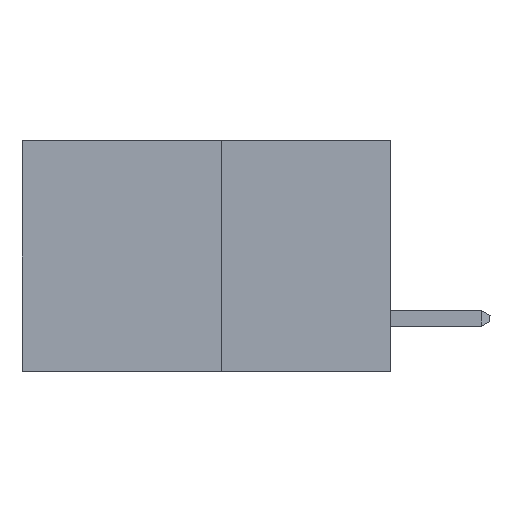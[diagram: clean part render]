
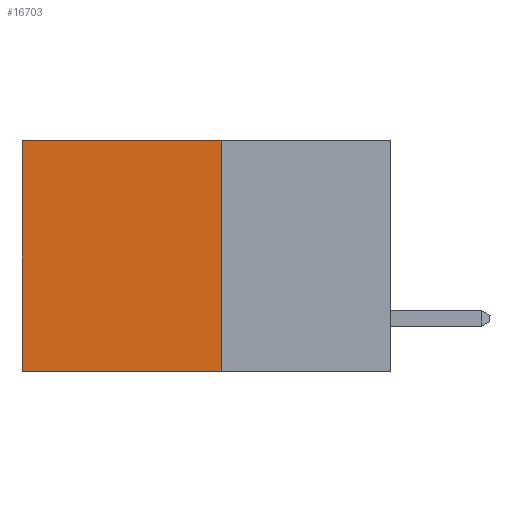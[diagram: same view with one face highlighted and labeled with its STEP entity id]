
A CAD part, left-side view. The second image highlights one B-rep face of the part: STEP entity #16703.
In plain terms, the highlighted planar face has unit normal (-1, 0, 0).
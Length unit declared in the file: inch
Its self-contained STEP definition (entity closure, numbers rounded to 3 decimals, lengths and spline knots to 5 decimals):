
#2117 = AXIS2_PLACEMENT_3D ( 'NONE', #9706, #24989, #11933 ) ;
#3600 = DIRECTION ( 'NONE',  ( 0., 1., 0. ) ) ;
#6845 = DIRECTION ( 'NONE',  ( 0., 1., 0. ) ) ;
#7923 = FACE_OUTER_BOUND ( 'NONE', #10808, .T. ) ;
#9315 = CARTESIAN_POINT ( 'NONE',  ( 0.277, 0.27, 0. ) ) ;
#9706 = CARTESIAN_POINT ( 'NONE',  ( 0.277, 0.27, -0.37 ) ) ;
#9708 = DIRECTION ( 'NONE',  ( 0., 0., -1. ) ) ;
#9910 = VERTEX_POINT ( 'NONE', #14942 ) ;
#10164 = VERTEX_POINT ( 'NONE', #13499 ) ;
#10249 = VERTEX_POINT ( 'NONE', #9315 ) ;
#10526 = ORIENTED_EDGE ( 'NONE', *, *, #21365, .F. ) ;
#10808 = EDGE_LOOP ( 'NONE', ( #26944, #21922, #10526, #20670 ) ) ;
#11181 = CARTESIAN_POINT ( 'NONE',  ( 0.277, 0.27, 0. ) ) ;
#11933 = DIRECTION ( 'NONE',  ( 0., 0., -1. ) ) ;
#12423 = CARTESIAN_POINT ( 'NONE',  ( 0.277, 0.27, -0.37 ) ) ;
#13499 = CARTESIAN_POINT ( 'NONE',  ( 0.277, 0.59, -0.37 ) ) ;
#13893 = VECTOR ( 'NONE', #15417, 39.37008 ) ;
#14040 = LINE ( 'NONE', #11181, #19149 ) ;
#14098 = EDGE_CURVE ( 'NONE', #10249, #9910, #14040, .T. ) ;
#14425 = EDGE_CURVE ( 'NONE', #18244, #10164, #16067, .T. ) ;
#14942 = CARTESIAN_POINT ( 'NONE',  ( 0.277, 0.59, 0. ) ) ;
#15417 = DIRECTION ( 'NONE',  ( 0., 0., -1. ) ) ;
#16067 = LINE ( 'NONE', #16719, #17435 ) ;
#16703 = ADVANCED_FACE ( 'NONE', ( #7923 ), #18351, .F. ) ;
#16719 = CARTESIAN_POINT ( 'NONE',  ( 0.277, 0.27, -0.37 ) ) ;
#17435 = VECTOR ( 'NONE', #3600, 39.37008 ) ;
#18244 = VERTEX_POINT ( 'NONE', #12423 ) ;
#18351 = PLANE ( 'NONE',  #2117 ) ;
#19149 = VECTOR ( 'NONE', #6845, 39.37008 ) ;
#19673 = LINE ( 'NONE', #26152, #13893 ) ;
#20670 = ORIENTED_EDGE ( 'NONE', *, *, #14098, .T. ) ;
#21365 = EDGE_CURVE ( 'NONE', #10249, #18244, #19673, .T. ) ;
#21922 = ORIENTED_EDGE ( 'NONE', *, *, #14425, .F. ) ;
#22805 = CARTESIAN_POINT ( 'NONE',  ( 0.277, 0.59, -0.37 ) ) ;
#23748 = EDGE_CURVE ( 'NONE', #9910, #10164, #26850, .T. ) ;
#24989 = DIRECTION ( 'NONE',  ( 1., 0., 0. ) ) ;
#26152 = CARTESIAN_POINT ( 'NONE',  ( 0.277, 0.27, -0.37 ) ) ;
#26850 = LINE ( 'NONE', #22805, #28191 ) ;
#26944 = ORIENTED_EDGE ( 'NONE', *, *, #23748, .T. ) ;
#28191 = VECTOR ( 'NONE', #9708, 39.37008 ) ;
